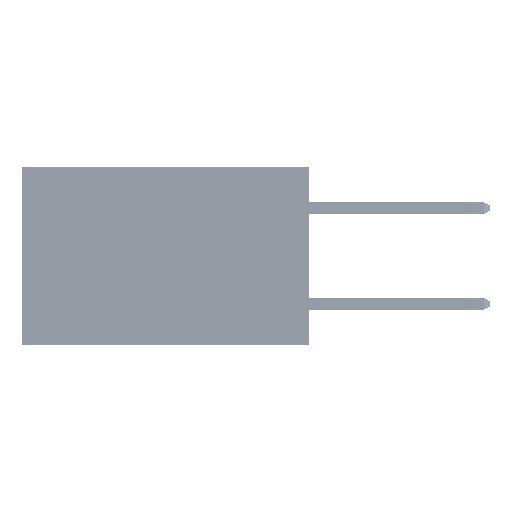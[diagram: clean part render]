
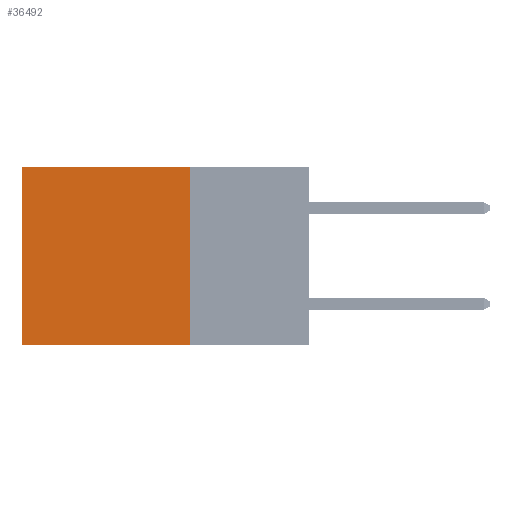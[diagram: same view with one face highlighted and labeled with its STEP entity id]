
A CAD part, left-side view. The second image highlights one B-rep face of the part: STEP entity #36492.
In plain terms, the highlighted planar face has unit normal (-1, 0, 0).
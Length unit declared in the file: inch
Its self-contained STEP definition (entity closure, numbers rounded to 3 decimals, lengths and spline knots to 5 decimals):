
#1491 = LINE ( 'NONE', #38133, #24636 ) ;
#3210 = ORIENTED_EDGE ( 'NONE', *, *, #24489, .T. ) ;
#5038 = DIRECTION ( 'NONE',  ( 0., 0., -1. ) ) ;
#6031 = DIRECTION ( 'NONE',  ( 0., 0., -1. ) ) ;
#7233 = AXIS2_PLACEMENT_3D ( 'NONE', #36871, #20918, #5038 ) ;
#8530 = EDGE_CURVE ( 'NONE', #49038, #39166, #12851, .T. ) ;
#12791 = CARTESIAN_POINT ( 'NONE',  ( 0.2875, 0.25, -0.37 ) ) ;
#12851 = LINE ( 'NONE', #21225, #21945 ) ;
#16203 = EDGE_CURVE ( 'NONE', #39166, #40964, #24475, .T. ) ;
#16694 = DIRECTION ( 'NONE',  ( 0., 1., 0. ) ) ;
#17173 = PLANE ( 'NONE',  #7233 ) ;
#17465 = VERTEX_POINT ( 'NONE', #20114 ) ;
#20020 = CARTESIAN_POINT ( 'NONE',  ( 0.2875, 0.25, -0.37 ) ) ;
#20114 = CARTESIAN_POINT ( 'NONE',  ( 0.2875, 0.6, 0. ) ) ;
#20918 = DIRECTION ( 'NONE',  ( 1., 0., 0. ) ) ;
#21225 = CARTESIAN_POINT ( 'NONE',  ( 0.2875, 0.25, 0. ) ) ;
#21945 = VECTOR ( 'NONE', #6031, 39.37008 ) ;
#21997 = DIRECTION ( 'NONE',  ( 0., 1., 0. ) ) ;
#24475 = LINE ( 'NONE', #12791, #48931 ) ;
#24489 = EDGE_CURVE ( 'NONE', #49038, #17465, #1491, .T. ) ;
#24636 = VECTOR ( 'NONE', #21997, 39.37008 ) ;
#26748 = CARTESIAN_POINT ( 'NONE',  ( 0.2875, 0.25, 0. ) ) ;
#26792 = CARTESIAN_POINT ( 'NONE',  ( 0.2875, 0.6, 0. ) ) ;
#29516 = EDGE_LOOP ( 'NONE', ( #32039, #35874, #36255, #3210 ) ) ;
#30849 = CARTESIAN_POINT ( 'NONE',  ( 0.2875, 0.6, -0.37 ) ) ;
#31158 = VECTOR ( 'NONE', #42529, 39.37008 ) ;
#32039 = ORIENTED_EDGE ( 'NONE', *, *, #38429, .T. ) ;
#35874 = ORIENTED_EDGE ( 'NONE', *, *, #16203, .F. ) ;
#36255 = ORIENTED_EDGE ( 'NONE', *, *, #8530, .F. ) ;
#36492 = ADVANCED_FACE ( 'NONE', ( #49126 ), #17173, .F. ) ;
#36871 = CARTESIAN_POINT ( 'NONE',  ( 0.2875, 0.25, 0. ) ) ;
#38133 = CARTESIAN_POINT ( 'NONE',  ( 0.2875, 0.25, 0. ) ) ;
#38429 = EDGE_CURVE ( 'NONE', #17465, #40964, #49511, .T. ) ;
#39166 = VERTEX_POINT ( 'NONE', #20020 ) ;
#40964 = VERTEX_POINT ( 'NONE', #30849 ) ;
#42529 = DIRECTION ( 'NONE',  ( 0., 0., -1. ) ) ;
#48931 = VECTOR ( 'NONE', #16694, 39.37008 ) ;
#49038 = VERTEX_POINT ( 'NONE', #26748 ) ;
#49126 = FACE_OUTER_BOUND ( 'NONE', #29516, .T. ) ;
#49511 = LINE ( 'NONE', #26792, #31158 ) ;
